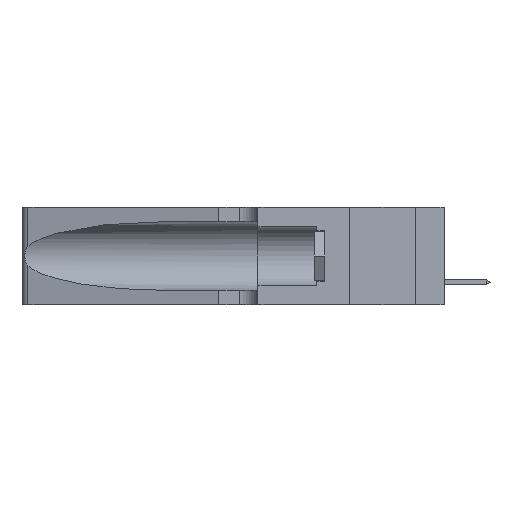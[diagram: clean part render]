
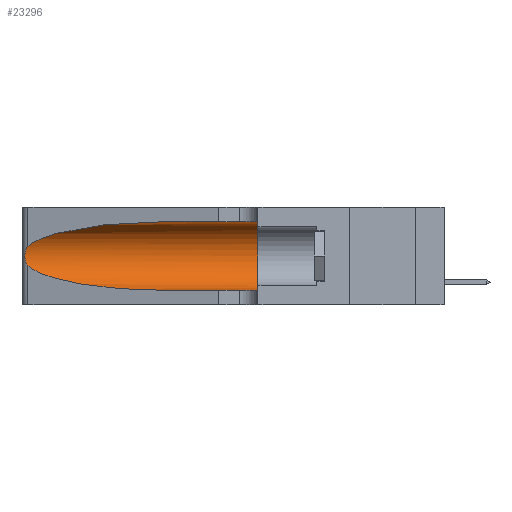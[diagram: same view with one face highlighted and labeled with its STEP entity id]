
A CAD part, left-side view. The second image highlights one B-rep face of the part: STEP entity #23296.
In plain terms, the highlighted cylindrical face has radius 3.308 mm (diameter 6.617 mm), a partial arc.
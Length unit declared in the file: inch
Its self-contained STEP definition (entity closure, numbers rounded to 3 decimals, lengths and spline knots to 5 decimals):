
#347 = VERTEX_POINT ( 'NONE', #21867 ) ;
#1529 = CARTESIAN_POINT ( 'NONE',  ( 0.26075, 1.23896, 0.178 ) ) ;
#1745 = CARTESIAN_POINT ( 'NONE',  ( 0.25789, 1.23486, 0.15765 ) ) ;
#1834 = VERTEX_POINT ( 'NONE', #21369 ) ;
#2279 = VERTEX_POINT ( 'NONE', #33608 ) ;
#2534 = FACE_OUTER_BOUND ( 'NONE', #8859, .T. ) ;
#2741 = ORIENTED_EDGE ( 'NONE', *, *, #20055, .T. ) ;
#4076 = DIRECTION ( 'NONE',  ( 0., 1., 0. ) ) ;
#4212 = VECTOR ( 'NONE', #10425, 39.37008 ) ;
#4611 = CARTESIAN_POINT ( 'NONE',  ( 0.25639, 1.23186, 0.15144 ) ) ;
#4859 = CARTESIAN_POINT ( 'NONE',  ( 0.25487, 1.22718, 0.14631 ) ) ;
#4860 = B_SPLINE_CURVE_WITH_KNOTS ( 'NONE', 3,
 ( #11744, #14029, #16888, #24786, #30073, #33068, #25569, #1529, #15042, #30319, #1745, #4611, #9538, #25117 ),
 .UNSPECIFIED., .F., .F.,
 ( 4, 2, 2, 2, 2, 2, 4 ),
 ( 0., 0.00027, 0.00053, 0.00107, 0.0016, 0.00187, 0.00214 ),
 .UNSPECIFIED. ) ;
#5795 = ORIENTED_EDGE ( 'NONE', *, *, #31433, .T. ) ;
#7475 = CARTESIAN_POINT ( 'NONE',  ( 0.1305, 0.72297, 0.31525 ) ) ;
#8473 = CARTESIAN_POINT ( 'NONE',  ( 0.1305, 0.72297, 0.05475 ) ) ;
#8716 = ORIENTED_EDGE ( 'NONE', *, *, #10381, .T. ) ;
#8859 = EDGE_LOOP ( 'NONE', ( #16031, #5795, #2741, #8716, #10120, #12472 ) ) ;
#9325 = DIRECTION ( 'NONE',  ( 0., 0., 1. ) ) ;
#9538 = CARTESIAN_POINT ( 'NONE',  ( 0.25555, 1.22993, 0.14849 ) ) ;
#10120 = ORIENTED_EDGE ( 'NONE', *, *, #27277, .F. ) ;
#10174 = AXIS2_PLACEMENT_3D ( 'NONE', #33184, #4076, #9325 ) ;
#10308 = CARTESIAN_POINT ( 'NONE',  ( 0.1305, 1.61858, 0.05475 ) ) ;
#10381 = EDGE_CURVE ( 'NONE', #25519, #2279, #26775, .T. ) ;
#10425 = DIRECTION ( 'NONE',  ( 0., -1., 0. ) ) ;
#11664 = CARTESIAN_POINT ( 'NONE',  ( 0.25487, 1.22718, 0.22369 ) ) ;
#11744 = CARTESIAN_POINT ( 'NONE',  ( 0.25487, 1.22718, 0.22369 ) ) ;
#11929 = LINE ( 'NONE', #17281, #25858 ) ;
#12472 = ORIENTED_EDGE ( 'NONE', *, *, #23945, .F. ) ;
#12779 = CARTESIAN_POINT ( 'NONE',  ( 0.1305, 0.72297, 0.05475 ) ) ;
#14029 = CARTESIAN_POINT ( 'NONE',  ( 0.25555, 1.22994, 0.2215 ) ) ;
#14524 =( BOUNDED_CURVE ( )  B_SPLINE_CURVE ( 3, ( #4859, #33641, #23420, #12779 ),
 .UNSPECIFIED., .F., .F. ) 
 B_SPLINE_CURVE_WITH_KNOTS ( ( 4, 4 ),
 ( 3.44316, 4.71239 ),
 .UNSPECIFIED. ) 
 CURVE ( )  GEOMETRIC_REPRESENTATION_ITEM ( )  RATIONAL_B_SPLINE_CURVE ( ( 1., 0.87, 0.87, 1. ) ) 
 REPRESENTATION_ITEM ( '' )  );
#15042 = CARTESIAN_POINT ( 'NONE',  ( 0.26017, 1.23833, 0.17102 ) ) ;
#16031 = ORIENTED_EDGE ( 'NONE', *, *, #32670, .T. ) ;
#16588 = CARTESIAN_POINT ( 'NONE',  ( 0.18966, 0.96281, 0.31525 ) ) ;
#16714 = CARTESIAN_POINT ( 'NONE',  ( 0.2373, 1.15595, 0.28018 ) ) ;
#16888 = CARTESIAN_POINT ( 'NONE',  ( 0.25639, 1.23184, 0.21858 ) ) ;
#17281 = CARTESIAN_POINT ( 'NONE',  ( 0.1305, 1.61858, 0.31525 ) ) ;
#20037 = DIRECTION ( 'NONE',  ( 0., -1., 0. ) ) ;
#20055 = EDGE_CURVE ( 'NONE', #33275, #25519, #14524, .T. ) ;
#21016 = CIRCLE ( 'NONE', #10174, 0.13025 ) ;
#21369 = CARTESIAN_POINT ( 'NONE',  ( 0.1305, 0.35, 0.31525 ) ) ;
#21716 = CARTESIAN_POINT ( 'NONE',  ( 0.25487, 1.22718, 0.14631 ) ) ;
#21867 = CARTESIAN_POINT ( 'NONE',  ( 0.25487, 1.22718, 0.22369 ) ) ;
#22646 = CYLINDRICAL_SURFACE ( 'NONE', #32941, 0.13025 ) ;
#23296 = ADVANCED_FACE ( 'NONE', ( #2534 ), #22646, .F. ) ;
#23420 = CARTESIAN_POINT ( 'NONE',  ( 0.18966, 0.96281, 0.05475 ) ) ;
#23945 = EDGE_CURVE ( 'NONE', #33642, #1834, #11929, .T. ) ;
#24786 = CARTESIAN_POINT ( 'NONE',  ( 0.25787, 1.23484, 0.2124 ) ) ;
#24884 = DIRECTION ( 'NONE',  ( 0., 0., -1. ) ) ;
#25117 = CARTESIAN_POINT ( 'NONE',  ( 0.25487, 1.22718, 0.14631 ) ) ;
#25519 = VERTEX_POINT ( 'NONE', #8473 ) ;
#25569 = CARTESIAN_POINT ( 'NONE',  ( 0.26075, 1.23896, 0.19203 ) ) ;
#25858 = VECTOR ( 'NONE', #20037, 39.37008 ) ;
#26775 = LINE ( 'NONE', #10308, #4212 ) ;
#27277 = EDGE_CURVE ( 'NONE', #1834, #2279, #21016, .T. ) ;
#27856 = CARTESIAN_POINT ( 'NONE',  ( 0.1305, 1.61858, 0.185 ) ) ;
#29554 = CARTESIAN_POINT ( 'NONE',  ( 0.1305, 0.72297, 0.31525 ) ) ;
#30073 = CARTESIAN_POINT ( 'NONE',  ( 0.25854, 1.2359, 0.20912 ) ) ;
#30166 = DIRECTION ( 'NONE',  ( 0., -1., 0. ) ) ;
#30319 = CARTESIAN_POINT ( 'NONE',  ( 0.25856, 1.23593, 0.16098 ) ) ;
#31433 = EDGE_CURVE ( 'NONE', #347, #33275, #4860, .T. ) ;
#32670 = EDGE_CURVE ( 'NONE', #33642, #347, #32831, .T. ) ;
#32831 =( BOUNDED_CURVE ( )  B_SPLINE_CURVE ( 3, ( #29554, #16588, #16714, #11664 ),
 .UNSPECIFIED., .F., .F. ) 
 B_SPLINE_CURVE_WITH_KNOTS ( ( 4, 4 ),
 ( 1.5708, 2.84003 ),
 .UNSPECIFIED. ) 
 CURVE ( )  GEOMETRIC_REPRESENTATION_ITEM ( )  RATIONAL_B_SPLINE_CURVE ( ( 1., 0.87, 0.87, 1. ) ) 
 REPRESENTATION_ITEM ( '' )  );
#32941 = AXIS2_PLACEMENT_3D ( 'NONE', #27856, #30166, #24884 ) ;
#33068 = CARTESIAN_POINT ( 'NONE',  ( 0.26018, 1.23835, 0.19895 ) ) ;
#33184 = CARTESIAN_POINT ( 'NONE',  ( 0.1305, 0.35, 0.185 ) ) ;
#33275 = VERTEX_POINT ( 'NONE', #21716 ) ;
#33608 = CARTESIAN_POINT ( 'NONE',  ( 0.1305, 0.35, 0.05475 ) ) ;
#33641 = CARTESIAN_POINT ( 'NONE',  ( 0.2373, 1.15595, 0.08982 ) ) ;
#33642 = VERTEX_POINT ( 'NONE', #7475 ) ;
